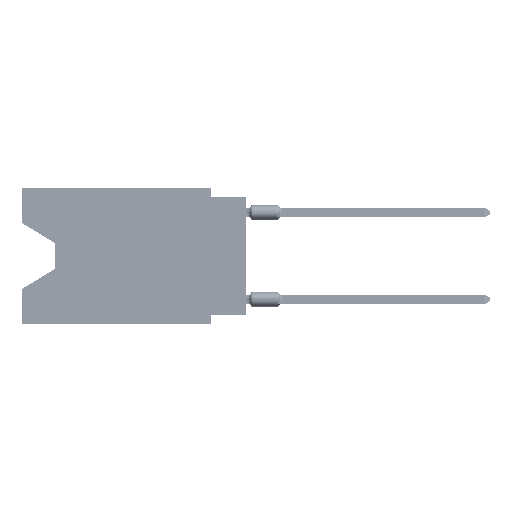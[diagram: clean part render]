
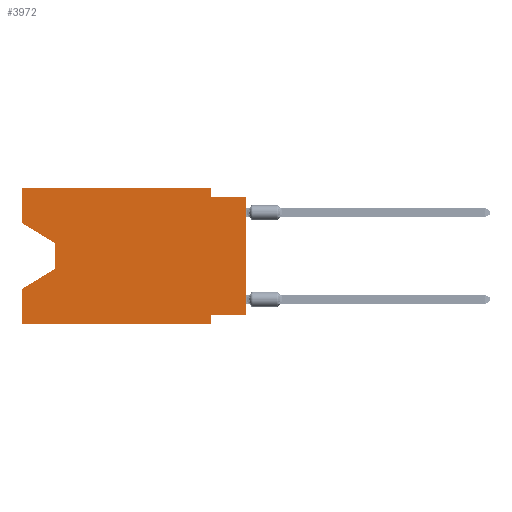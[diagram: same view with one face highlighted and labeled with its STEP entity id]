
A CAD part, left-side view. The second image highlights one B-rep face of the part: STEP entity #3972.
In plain terms, the highlighted planar face has unit normal (-1, 0, 0).
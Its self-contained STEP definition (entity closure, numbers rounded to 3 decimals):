
#1006 = CARTESIAN_POINT ( 'NONE',  ( 0., 16.383, -9.906 ) ) ;
#1378 = CARTESIAN_POINT ( 'NONE',  ( 0., 16.383, 0. ) ) ;
#1925 = VECTOR ( 'NONE', #4215, 1000. ) ;
#2172 = CARTESIAN_POINT ( 'NONE',  ( 0., 16.383, -2.546 ) ) ;
#3972 = ADVANCED_FACE ( 'NONE', ( #9105 ), #4852, .F. ) ;
#4215 = DIRECTION ( 'NONE',  ( 0., 0., 1. ) ) ;
#4309 = CARTESIAN_POINT ( 'NONE',  ( 0., 2.54, 0. ) ) ;
#4852 = PLANE ( 'NONE',  #15516 ) ;
#6143 = VECTOR ( 'NONE', #52544, 1000. ) ;
#7110 = VERTEX_POINT ( 'NONE', #51416 ) ;
#8674 = LINE ( 'NONE', #20598, #58381 ) ;
#9105 = FACE_OUTER_BOUND ( 'NONE', #69991, .T. ) ;
#12130 = CARTESIAN_POINT ( 'NONE',  ( 0., 13.97, -4.013 ) ) ;
#15516 = AXIS2_PLACEMENT_3D ( 'NONE', #21404, #21792, #28331 ) ;
#16341 = LINE ( 'NONE', #57544, #27012 ) ;
#16780 = CARTESIAN_POINT ( 'NONE',  ( 0., 2.54, -9.271 ) ) ;
#19060 = VECTOR ( 'NONE', #51289, 1000. ) ;
#19118 = VECTOR ( 'NONE', #69079, 1000. ) ;
#19419 = ORIENTED_EDGE ( 'NONE', *, *, #23424, .F. ) ;
#19853 = DIRECTION ( 'NONE',  ( 0., 0.855, -0.519 ) ) ;
#20324 = EDGE_CURVE ( 'NONE', #75094, #26221, #8674, .T. ) ;
#20598 = CARTESIAN_POINT ( 'NONE',  ( 0., 13.97, -5.893 ) ) ;
#20862 = LINE ( 'NONE', #4309, #19060 ) ;
#21404 = CARTESIAN_POINT ( 'NONE',  ( 0., 16.383, 0. ) ) ;
#21411 = VERTEX_POINT ( 'NONE', #56199 ) ;
#21567 = DIRECTION ( 'NONE',  ( 0., 0., 1. ) ) ;
#21792 = DIRECTION ( 'NONE',  ( 1., 0., 0. ) ) ;
#21980 = ORIENTED_EDGE ( 'NONE', *, *, #49997, .F. ) ;
#22127 = CARTESIAN_POINT ( 'NONE',  ( 0., 16.383, -9.906 ) ) ;
#22354 = ORIENTED_EDGE ( 'NONE', *, *, #69718, .T. ) ;
#23152 = DIRECTION ( 'NONE',  ( 0., 1., 0. ) ) ;
#23424 = EDGE_CURVE ( 'NONE', #7110, #51783, #20862, .T. ) ;
#23571 = CARTESIAN_POINT ( 'NONE',  ( 0., 13.97, -5.893 ) ) ;
#23718 = DIRECTION ( 'NONE',  ( 0., -1., 0. ) ) ;
#23913 = EDGE_CURVE ( 'NONE', #29963, #26221, #73129, .T. ) ;
#25039 = VERTEX_POINT ( 'NONE', #16780 ) ;
#25241 = VECTOR ( 'NONE', #23152, 1000. ) ;
#26221 = VERTEX_POINT ( 'NONE', #74265 ) ;
#26944 = CARTESIAN_POINT ( 'NONE',  ( 0., 16.383, 0. ) ) ;
#27012 = VECTOR ( 'NONE', #58314, 1000. ) ;
#27880 = LINE ( 'NONE', #70211, #41566 ) ;
#28331 = DIRECTION ( 'NONE',  ( 0., 0., -1. ) ) ;
#29435 = CARTESIAN_POINT ( 'NONE',  ( 0., 13.97, -4.013 ) ) ;
#29549 = ORIENTED_EDGE ( 'NONE', *, *, #20324, .T. ) ;
#29655 = EDGE_CURVE ( 'NONE', #51783, #75077, #48753, .T. ) ;
#29963 = VERTEX_POINT ( 'NONE', #22127 ) ;
#32759 = LINE ( 'NONE', #68158, #49437 ) ;
#32967 = ORIENTED_EDGE ( 'NONE', *, *, #23913, .F. ) ;
#34055 = CARTESIAN_POINT ( 'NONE',  ( 0., 16.383, -2.546 ) ) ;
#34064 = EDGE_CURVE ( 'NONE', #46517, #35945, #32759, .T. ) ;
#34816 = ORIENTED_EDGE ( 'NONE', *, *, #50090, .T. ) ;
#34874 = EDGE_CURVE ( 'NONE', #35945, #7110, #54499, .T. ) ;
#35945 = VERTEX_POINT ( 'NONE', #40398 ) ;
#39187 = VECTOR ( 'NONE', #47999, 1000. ) ;
#40398 = CARTESIAN_POINT ( 'NONE',  ( 0., 16.383, 0. ) ) ;
#41438 = DIRECTION ( 'NONE',  ( 0., -1., 0. ) ) ;
#41566 = VECTOR ( 'NONE', #51370, 1000. ) ;
#41634 = CARTESIAN_POINT ( 'NONE',  ( 0., 0., -9.271 ) ) ;
#42941 = ORIENTED_EDGE ( 'NONE', *, *, #29655, .F. ) ;
#45616 = LINE ( 'NONE', #34055, #19118 ) ;
#45694 = VERTEX_POINT ( 'NONE', #67767 ) ;
#46517 = VERTEX_POINT ( 'NONE', #2172 ) ;
#47904 = LINE ( 'NONE', #29435, #6143 ) ;
#47999 = DIRECTION ( 'NONE',  ( 0., -1., 0. ) ) ;
#48574 = CARTESIAN_POINT ( 'NONE',  ( 0., 0., -0.635 ) ) ;
#48753 = LINE ( 'NONE', #60686, #39187 ) ;
#49437 = VECTOR ( 'NONE', #21567, 1000. ) ;
#49997 = EDGE_CURVE ( 'NONE', #25039, #45694, #16341, .T. ) ;
#50090 = EDGE_CURVE ( 'NONE', #67025, #75094, #47904, .T. ) ;
#51289 = DIRECTION ( 'NONE',  ( 0., 0., -1. ) ) ;
#51370 = DIRECTION ( 'NONE',  ( 0., 0., 1. ) ) ;
#51416 = CARTESIAN_POINT ( 'NONE',  ( 0., 2.54, 0. ) ) ;
#51783 = VERTEX_POINT ( 'NONE', #61661 ) ;
#52024 = VECTOR ( 'NONE', #23718, 1000. ) ;
#52544 = DIRECTION ( 'NONE',  ( 0., 0., -1. ) ) ;
#53748 = LINE ( 'NONE', #1006, #58061 ) ;
#54499 = LINE ( 'NONE', #1378, #52024 ) ;
#54771 = ORIENTED_EDGE ( 'NONE', *, *, #34874, .F. ) ;
#56199 = CARTESIAN_POINT ( 'NONE',  ( 0., 0., -9.271 ) ) ;
#57335 = EDGE_CURVE ( 'NONE', #29963, #45694, #53748, .T. ) ;
#57544 = CARTESIAN_POINT ( 'NONE',  ( 0., 2.54, -9.906 ) ) ;
#58061 = VECTOR ( 'NONE', #41438, 1000. ) ;
#58212 = LINE ( 'NONE', #41634, #25241 ) ;
#58314 = DIRECTION ( 'NONE',  ( 0., 0., -1. ) ) ;
#58381 = VECTOR ( 'NONE', #19853, 1000. ) ;
#60686 = CARTESIAN_POINT ( 'NONE',  ( 0., 0., -0.635 ) ) ;
#61661 = CARTESIAN_POINT ( 'NONE',  ( 0., 2.54, -0.635 ) ) ;
#62238 = EDGE_CURVE ( 'NONE', #21411, #25039, #58212, .T. ) ;
#63181 = EDGE_CURVE ( 'NONE', #46517, #67025, #45616, .T. ) ;
#67025 = VERTEX_POINT ( 'NONE', #12130 ) ;
#67767 = CARTESIAN_POINT ( 'NONE',  ( 0., 2.54, -9.906 ) ) ;
#68158 = CARTESIAN_POINT ( 'NONE',  ( 0., 16.383, 0. ) ) ;
#68272 = ORIENTED_EDGE ( 'NONE', *, *, #63181, .T. ) ;
#69079 = DIRECTION ( 'NONE',  ( 0., -0.855, -0.519 ) ) ;
#69531 = ORIENTED_EDGE ( 'NONE', *, *, #34064, .F. ) ;
#69718 = EDGE_CURVE ( 'NONE', #21411, #75077, #27880, .T. ) ;
#69991 = EDGE_LOOP ( 'NONE', ( #68272, #34816, #29549, #32967, #72605, #21980, #75151, #22354, #42941, #19419, #54771, #69531 ) ) ;
#70211 = CARTESIAN_POINT ( 'NONE',  ( 0., 0., 0. ) ) ;
#72605 = ORIENTED_EDGE ( 'NONE', *, *, #57335, .T. ) ;
#73129 = LINE ( 'NONE', #26944, #1925 ) ;
#74265 = CARTESIAN_POINT ( 'NONE',  ( 0., 16.383, -7.36 ) ) ;
#75077 = VERTEX_POINT ( 'NONE', #48574 ) ;
#75094 = VERTEX_POINT ( 'NONE', #23571 ) ;
#75151 = ORIENTED_EDGE ( 'NONE', *, *, #62238, .F. ) ;
